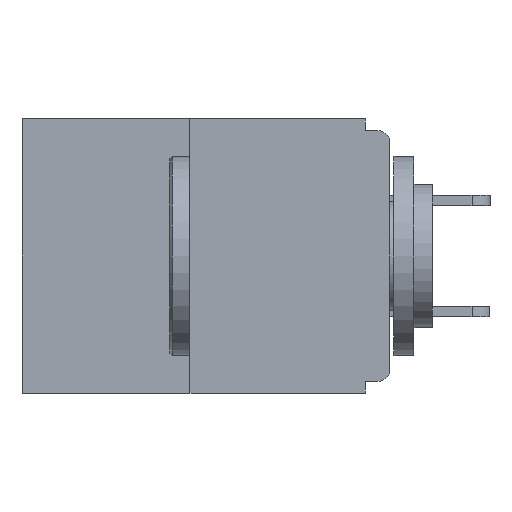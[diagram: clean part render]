
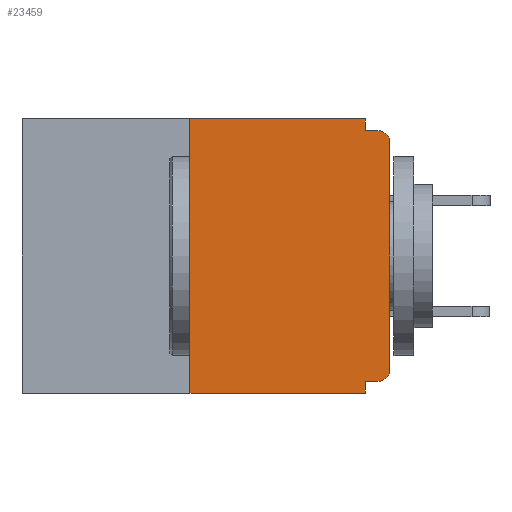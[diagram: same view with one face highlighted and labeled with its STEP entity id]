
A CAD part, left-side view. The second image highlights one B-rep face of the part: STEP entity #23459.
In plain terms, the highlighted planar face has unit normal (-1, 0, 0).
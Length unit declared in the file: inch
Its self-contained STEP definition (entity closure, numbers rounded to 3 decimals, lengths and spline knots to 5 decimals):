
#8 = EDGE_CURVE ( 'NONE', #22522, #17728, #19861, .T. ) ;
#74 = CARTESIAN_POINT ( 'NONE',  ( 0., 0.031, -0.343 ) ) ;
#571 = FACE_OUTER_BOUND ( 'NONE', #9429, .T. ) ;
#894 = AXIS2_PLACEMENT_3D ( 'NONE', #18820, #20877, #18905 ) ;
#956 = EDGE_CURVE ( 'NONE', #12742, #15599, #13085, .T. ) ;
#1356 = ORIENTED_EDGE ( 'NONE', *, *, #6509, .F. ) ;
#1405 = CARTESIAN_POINT ( 'NONE',  ( 0., 0.015, -0.015 ) ) ;
#1697 = ORIENTED_EDGE ( 'NONE', *, *, #9895, .F. ) ;
#1747 = VECTOR ( 'NONE', #4390, 39.37008 ) ;
#2220 = EDGE_CURVE ( 'NONE', #5974, #4233, #4762, .T. ) ;
#2222 = ORIENTED_EDGE ( 'NONE', *, *, #2220, .F. ) ;
#2461 = CARTESIAN_POINT ( 'NONE',  ( 0., 0.46, 0. ) ) ;
#2539 = DIRECTION ( 'NONE',  ( 0., 0., -1. ) ) ;
#3042 = AXIS2_PLACEMENT_3D ( 'NONE', #2461, #6361, #2539 ) ;
#3699 = CARTESIAN_POINT ( 'NONE',  ( 0., 0.031, 0. ) ) ;
#4030 = DIRECTION ( 'NONE',  ( 0., -1., 0. ) ) ;
#4233 = VERTEX_POINT ( 'NONE', #21690 ) ;
#4390 = DIRECTION ( 'NONE',  ( 0., 0., 1. ) ) ;
#4448 = VECTOR ( 'NONE', #24122, 39.37008 ) ;
#4762 = LINE ( 'NONE', #6187, #19442 ) ;
#4822 = DIRECTION ( 'NONE',  ( -1., 0., 0. ) ) ;
#4833 = EDGE_CURVE ( 'NONE', #5974, #16782, #10296, .T. ) ;
#5235 = DIRECTION ( 'NONE',  ( 0., -1., 0. ) ) ;
#5266 = VERTEX_POINT ( 'NONE', #1405 ) ;
#5756 = ORIENTED_EDGE ( 'NONE', *, *, #956, .F. ) ;
#5974 = VERTEX_POINT ( 'NONE', #20739 ) ;
#6004 = ORIENTED_EDGE ( 'NONE', *, *, #4833, .T. ) ;
#6131 = VECTOR ( 'NONE', #5235, 39.37008 ) ;
#6187 = CARTESIAN_POINT ( 'NONE',  ( 0., 0., -0.328 ) ) ;
#6361 = DIRECTION ( 'NONE',  ( 1., 0., 0. ) ) ;
#6509 = EDGE_CURVE ( 'NONE', #23582, #5266, #9650, .T. ) ;
#6569 = VECTOR ( 'NONE', #20702, 39.37008 ) ;
#6593 = EDGE_CURVE ( 'NONE', #16782, #13507, #14813, .T. ) ;
#6598 = CARTESIAN_POINT ( 'NONE',  ( 0., 0., 0. ) ) ;
#6866 = CIRCLE ( 'NONE', #894, 0.015 ) ;
#7066 = LINE ( 'NONE', #74, #18373 ) ;
#7811 = LINE ( 'NONE', #20775, #6569 ) ;
#7873 = CARTESIAN_POINT ( 'NONE',  ( 0., 0.031, -0.343 ) ) ;
#9421 = ORIENTED_EDGE ( 'NONE', *, *, #8, .T. ) ;
#9429 = EDGE_LOOP ( 'NONE', ( #5756, #9445, #9421, #1697, #2222, #6004, #15077, #11541, #1356, #19876 ) ) ;
#9445 = ORIENTED_EDGE ( 'NONE', *, *, #20638, .F. ) ;
#9650 = LINE ( 'NONE', #20341, #4448 ) ;
#9793 = VECTOR ( 'NONE', #4030, 39.37008 ) ;
#9895 = EDGE_CURVE ( 'NONE', #4233, #17728, #7066, .T. ) ;
#10296 = CIRCLE ( 'NONE', #14283, 0.015 ) ;
#11541 = ORIENTED_EDGE ( 'NONE', *, *, #13326, .T. ) ;
#12144 = CARTESIAN_POINT ( 'NONE',  ( 0., 0.25, -0.343 ) ) ;
#12742 = VERTEX_POINT ( 'NONE', #18225 ) ;
#13085 = LINE ( 'NONE', #25142, #6131 ) ;
#13326 = EDGE_CURVE ( 'NONE', #13507, #5266, #6866, .T. ) ;
#13507 = VERTEX_POINT ( 'NONE', #24623 ) ;
#14147 = CARTESIAN_POINT ( 'NONE',  ( 0., 0.46, -0.343 ) ) ;
#14283 = AXIS2_PLACEMENT_3D ( 'NONE', #20689, #4822, #22510 ) ;
#14813 = LINE ( 'NONE', #6598, #1747 ) ;
#15077 = ORIENTED_EDGE ( 'NONE', *, *, #6593, .T. ) ;
#15599 = VERTEX_POINT ( 'NONE', #18898 ) ;
#16496 = VECTOR ( 'NONE', #20641, 39.37008 ) ;
#16740 = CARTESIAN_POINT ( 'NONE',  ( 0., 0.031, -0.015 ) ) ;
#16782 = VERTEX_POINT ( 'NONE', #20312 ) ;
#17144 = LINE ( 'NONE', #3699, #16496 ) ;
#17728 = VERTEX_POINT ( 'NONE', #7873 ) ;
#17971 = DIRECTION ( 'NONE',  ( 0., 1., 0. ) ) ;
#18225 = CARTESIAN_POINT ( 'NONE',  ( 0., 0.25, 0. ) ) ;
#18373 = VECTOR ( 'NONE', #23568, 39.37008 ) ;
#18820 = CARTESIAN_POINT ( 'NONE',  ( 0., 0.015, -0.03 ) ) ;
#18898 = CARTESIAN_POINT ( 'NONE',  ( 0., 0.031, 0. ) ) ;
#18905 = DIRECTION ( 'NONE',  ( 0., 0., -1. ) ) ;
#19442 = VECTOR ( 'NONE', #17971, 39.37008 ) ;
#19861 = LINE ( 'NONE', #14147, #9793 ) ;
#19876 = ORIENTED_EDGE ( 'NONE', *, *, #21662, .F. ) ;
#20312 = CARTESIAN_POINT ( 'NONE',  ( 0., 0., -0.313 ) ) ;
#20341 = CARTESIAN_POINT ( 'NONE',  ( 0., 0., -0.015 ) ) ;
#20638 = EDGE_CURVE ( 'NONE', #22522, #12742, #7811, .T. ) ;
#20641 = DIRECTION ( 'NONE',  ( 0., 0., -1. ) ) ;
#20689 = CARTESIAN_POINT ( 'NONE',  ( 0., 0.015, -0.313 ) ) ;
#20702 = DIRECTION ( 'NONE',  ( 0., 0., 1. ) ) ;
#20739 = CARTESIAN_POINT ( 'NONE',  ( 0., 0.015, -0.328 ) ) ;
#20775 = CARTESIAN_POINT ( 'NONE',  ( 0., 0.25, 0. ) ) ;
#20877 = DIRECTION ( 'NONE',  ( -1., 0., 0. ) ) ;
#21662 = EDGE_CURVE ( 'NONE', #15599, #23582, #17144, .T. ) ;
#21690 = CARTESIAN_POINT ( 'NONE',  ( 0., 0.031, -0.328 ) ) ;
#22510 = DIRECTION ( 'NONE',  ( 0., 0., -1. ) ) ;
#22522 = VERTEX_POINT ( 'NONE', #12144 ) ;
#23459 = ADVANCED_FACE ( 'NONE', ( #571 ), #24047, .F. ) ;
#23568 = DIRECTION ( 'NONE',  ( 0., 0., -1. ) ) ;
#23582 = VERTEX_POINT ( 'NONE', #16740 ) ;
#24047 = PLANE ( 'NONE',  #3042 ) ;
#24122 = DIRECTION ( 'NONE',  ( 0., -1., 0. ) ) ;
#24623 = CARTESIAN_POINT ( 'NONE',  ( 0., 0., -0.03 ) ) ;
#25142 = CARTESIAN_POINT ( 'NONE',  ( 0., 0.46, 0. ) ) ;
